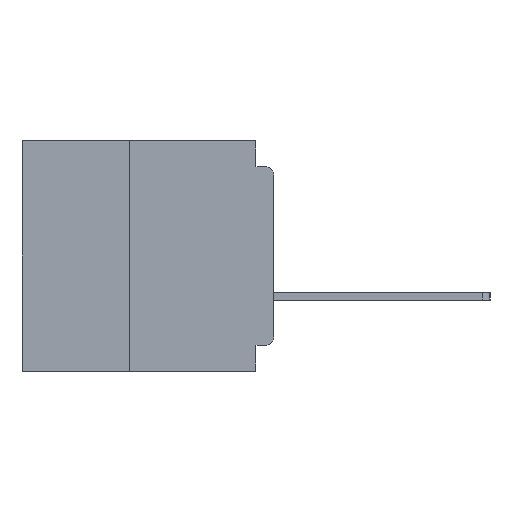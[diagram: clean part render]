
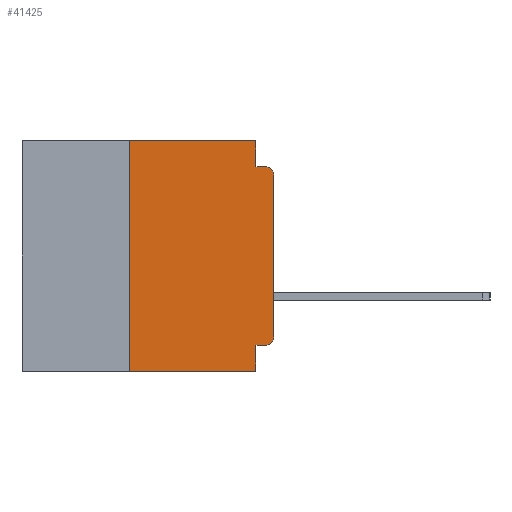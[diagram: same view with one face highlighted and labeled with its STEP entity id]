
A CAD part, left-side view. The second image highlights one B-rep face of the part: STEP entity #41425.
In plain terms, the highlighted planar face has unit normal (-1, 0, 0).
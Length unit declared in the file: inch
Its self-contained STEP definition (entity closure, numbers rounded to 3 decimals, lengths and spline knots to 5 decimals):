
#389 = CARTESIAN_POINT ( 'NONE',  ( 0., 0.015, -0.06 ) ) ;
#1821 = ORIENTED_EDGE ( 'NONE', *, *, #48862, .T. ) ;
#2059 = AXIS2_PLACEMENT_3D ( 'NONE', #389, #33332, #5148 ) ;
#2293 = VECTOR ( 'NONE', #2297, 39.37008 ) ;
#2297 = DIRECTION ( 'NONE',  ( 0., 0., -1. ) ) ;
#2402 = ORIENTED_EDGE ( 'NONE', *, *, #34142, .T. ) ;
#2998 = VECTOR ( 'NONE', #16590, 39.37008 ) ;
#3835 = LINE ( 'NONE', #46613, #16406 ) ;
#4347 = VECTOR ( 'NONE', #50126, 39.37008 ) ;
#4679 = ORIENTED_EDGE ( 'NONE', *, *, #25810, .T. ) ;
#5148 = DIRECTION ( 'NONE',  ( 0., 0., -1. ) ) ;
#5295 = VERTEX_POINT ( 'NONE', #24109 ) ;
#5978 = EDGE_CURVE ( 'NONE', #37978, #57552, #19324, .T. ) ;
#7490 = CARTESIAN_POINT ( 'NONE',  ( 0., 0.031, -0.4 ) ) ;
#7808 = VERTEX_POINT ( 'NONE', #7490 ) ;
#8108 = CIRCLE ( 'NONE', #2059, 0.015 ) ;
#8355 = DIRECTION ( 'NONE',  ( 0., 0., -1. ) ) ;
#10119 = EDGE_LOOP ( 'NONE', ( #60136, #2402, #13798, #32105, #24191, #14143, #1821, #35196, #11833, #4679 ) ) ;
#11119 = VECTOR ( 'NONE', #51812, 39.37008 ) ;
#11386 = EDGE_CURVE ( 'NONE', #47047, #45543, #3835, .T. ) ;
#11502 = CARTESIAN_POINT ( 'NONE',  ( 0., 0.031, -0.045 ) ) ;
#11817 = FACE_OUTER_BOUND ( 'NONE', #10119, .T. ) ;
#11833 = ORIENTED_EDGE ( 'NONE', *, *, #57653, .F. ) ;
#13737 = DIRECTION ( 'NONE',  ( 0., 0., 1. ) ) ;
#13798 = ORIENTED_EDGE ( 'NONE', *, *, #5978, .F. ) ;
#14143 = ORIENTED_EDGE ( 'NONE', *, *, #50645, .F. ) ;
#15096 = VERTEX_POINT ( 'NONE', #25608 ) ;
#16406 = VECTOR ( 'NONE', #13737, 39.37008 ) ;
#16590 = DIRECTION ( 'NONE',  ( 0., -1., 0. ) ) ;
#17262 = CARTESIAN_POINT ( 'NONE',  ( 0., 0., -0.355 ) ) ;
#17572 = CARTESIAN_POINT ( 'NONE',  ( 0., 0.25, 0. ) ) ;
#19281 = CARTESIAN_POINT ( 'NONE',  ( 0., 0.015, -0.34 ) ) ;
#19324 = LINE ( 'NONE', #28977, #55292 ) ;
#24004 = DIRECTION ( 'NONE',  ( 0., 0., -1. ) ) ;
#24109 = CARTESIAN_POINT ( 'NONE',  ( 0., 0.031, 0. ) ) ;
#24191 = ORIENTED_EDGE ( 'NONE', *, *, #24232, .F. ) ;
#24232 = EDGE_CURVE ( 'NONE', #30243, #5295, #28072, .T. ) ;
#25276 = CARTESIAN_POINT ( 'NONE',  ( 0., 0.015, -0.045 ) ) ;
#25608 = CARTESIAN_POINT ( 'NONE',  ( 0., 0.031, -0.355 ) ) ;
#25810 = EDGE_CURVE ( 'NONE', #29343, #47047, #52922, .T. ) ;
#26877 = PLANE ( 'NONE',  #28470 ) ;
#28072 = LINE ( 'NONE', #40036, #2998 ) ;
#28470 = AXIS2_PLACEMENT_3D ( 'NONE', #55165, #36514, #8355 ) ;
#28579 = VECTOR ( 'NONE', #37259, 39.37008 ) ;
#28977 = CARTESIAN_POINT ( 'NONE',  ( 0., 0., -0.045 ) ) ;
#29343 = VERTEX_POINT ( 'NONE', #43777 ) ;
#30014 = LINE ( 'NONE', #60818, #28579 ) ;
#30243 = VERTEX_POINT ( 'NONE', #17572 ) ;
#30614 = AXIS2_PLACEMENT_3D ( 'NONE', #19281, #52135, #24004 ) ;
#31458 = CARTESIAN_POINT ( 'NONE',  ( 0., 0., -0.06 ) ) ;
#32105 = ORIENTED_EDGE ( 'NONE', *, *, #34324, .F. ) ;
#32675 = CARTESIAN_POINT ( 'NONE',  ( 0., 0., -0.34 ) ) ;
#33332 = DIRECTION ( 'NONE',  ( -1., 0., 0. ) ) ;
#34142 = EDGE_CURVE ( 'NONE', #45543, #57552, #8108, .T. ) ;
#34324 = EDGE_CURVE ( 'NONE', #5295, #37978, #60223, .T. ) ;
#35196 = ORIENTED_EDGE ( 'NONE', *, *, #36818, .F. ) ;
#36514 = DIRECTION ( 'NONE',  ( 1., 0., 0. ) ) ;
#36818 = EDGE_CURVE ( 'NONE', #15096, #7808, #50895, .T. ) ;
#37259 = DIRECTION ( 'NONE',  ( 0., 0., 1. ) ) ;
#37627 = LINE ( 'NONE', #47096, #11119 ) ;
#37978 = VERTEX_POINT ( 'NONE', #11502 ) ;
#38412 = DIRECTION ( 'NONE',  ( 0., -1., 0. ) ) ;
#39300 = DIRECTION ( 'NONE',  ( 0., 0., -1. ) ) ;
#40036 = CARTESIAN_POINT ( 'NONE',  ( 0., 0.437, 0. ) ) ;
#41425 = ADVANCED_FACE ( 'NONE', ( #11817 ), #26877, .F. ) ;
#43777 = CARTESIAN_POINT ( 'NONE',  ( 0., 0.015, -0.355 ) ) ;
#43998 = CARTESIAN_POINT ( 'NONE',  ( 0., 0.031, 0. ) ) ;
#44493 = CARTESIAN_POINT ( 'NONE',  ( 0., 0.031, -0.4 ) ) ;
#45543 = VERTEX_POINT ( 'NONE', #31458 ) ;
#46317 = VECTOR ( 'NONE', #39300, 39.37008 ) ;
#46613 = CARTESIAN_POINT ( 'NONE',  ( 0., 0., 0. ) ) ;
#47047 = VERTEX_POINT ( 'NONE', #32675 ) ;
#47096 = CARTESIAN_POINT ( 'NONE',  ( 0., 0.437, -0.4 ) ) ;
#48862 = EDGE_CURVE ( 'NONE', #60955, #7808, #37627, .T. ) ;
#50126 = DIRECTION ( 'NONE',  ( 0., 1., 0. ) ) ;
#50645 = EDGE_CURVE ( 'NONE', #60955, #30243, #30014, .T. ) ;
#50895 = LINE ( 'NONE', #44493, #2293 ) ;
#51812 = DIRECTION ( 'NONE',  ( 0., -1., 0. ) ) ;
#52135 = DIRECTION ( 'NONE',  ( -1., 0., 0. ) ) ;
#52922 = CIRCLE ( 'NONE', #30614, 0.015 ) ;
#54392 = LINE ( 'NONE', #17262, #4347 ) ;
#55165 = CARTESIAN_POINT ( 'NONE',  ( 0., 0.437, 0. ) ) ;
#55292 = VECTOR ( 'NONE', #38412, 39.37008 ) ;
#57552 = VERTEX_POINT ( 'NONE', #25276 ) ;
#57653 = EDGE_CURVE ( 'NONE', #29343, #15096, #54392, .T. ) ;
#58756 = CARTESIAN_POINT ( 'NONE',  ( 0., 0.25, -0.4 ) ) ;
#60136 = ORIENTED_EDGE ( 'NONE', *, *, #11386, .T. ) ;
#60223 = LINE ( 'NONE', #43998, #46317 ) ;
#60818 = CARTESIAN_POINT ( 'NONE',  ( 0., 0.25, -0.4 ) ) ;
#60955 = VERTEX_POINT ( 'NONE', #58756 ) ;
